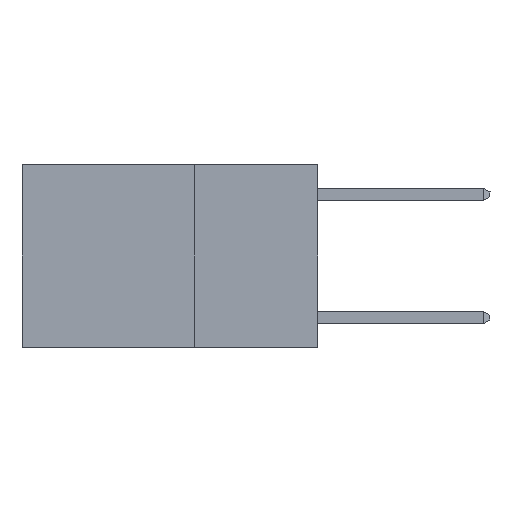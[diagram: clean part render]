
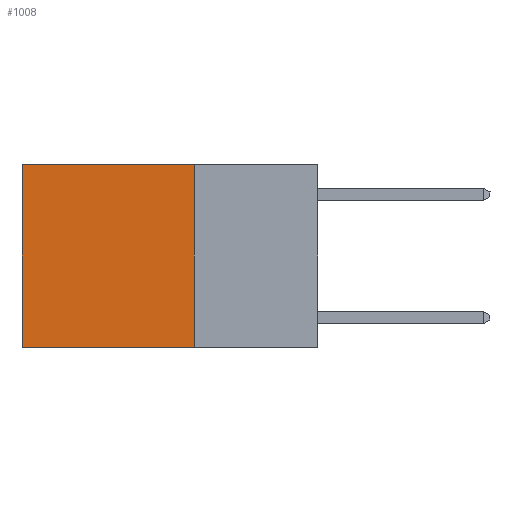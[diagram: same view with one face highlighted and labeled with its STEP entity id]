
A CAD part, left-side view. The second image highlights one B-rep face of the part: STEP entity #1008.
In plain terms, the highlighted planar face has unit normal (-1, 0, 0).
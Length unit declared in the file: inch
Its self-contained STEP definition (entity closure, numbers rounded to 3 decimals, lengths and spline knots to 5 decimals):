
#23 = ORIENTED_EDGE ( 'NONE', *, *, #8157, .T. ) ;
#970 = ORIENTED_EDGE ( 'NONE', *, *, #1598, .T. ) ;
#1008 = ADVANCED_FACE ( 'NONE', ( #7359 ), #7798, .F. ) ;
#1027 = LINE ( 'NONE', #3263, #15625 ) ;
#1598 = EDGE_CURVE ( 'NONE', #15399, #4673, #9685, .T. ) ;
#1655 = LINE ( 'NONE', #2238, #15828 ) ;
#2238 = CARTESIAN_POINT ( 'NONE',  ( 0.2625, 0.25, 0. ) ) ;
#2311 = CARTESIAN_POINT ( 'NONE',  ( 0.2625, 0.6, -0.37 ) ) ;
#2419 = DIRECTION ( 'NONE',  ( 0., 0., -1. ) ) ;
#3263 = CARTESIAN_POINT ( 'NONE',  ( 0.2625, 0.25, 0. ) ) ;
#4673 = VERTEX_POINT ( 'NONE', #2311 ) ;
#5084 = VECTOR ( 'NONE', #8416, 39.37008 ) ;
#5508 = LINE ( 'NONE', #9764, #5084 ) ;
#5667 = AXIS2_PLACEMENT_3D ( 'NONE', #12930, #12880, #9651 ) ;
#6391 = EDGE_LOOP ( 'NONE', ( #970, #12656, #12473, #23 ) ) ;
#6484 = CARTESIAN_POINT ( 'NONE',  ( 0.2625, 0.25, 0. ) ) ;
#6863 = VERTEX_POINT ( 'NONE', #14920 ) ;
#7359 = FACE_OUTER_BOUND ( 'NONE', #6391, .T. ) ;
#7798 = PLANE ( 'NONE',  #5667 ) ;
#7958 = EDGE_CURVE ( 'NONE', #13203, #6863, #1027, .T. ) ;
#8157 = EDGE_CURVE ( 'NONE', #13203, #15399, #1655, .T. ) ;
#8416 = DIRECTION ( 'NONE',  ( 0., 1., 0. ) ) ;
#8732 = DIRECTION ( 'NONE',  ( 0., 0., -1. ) ) ;
#9247 = CARTESIAN_POINT ( 'NONE',  ( 0.2625, 0.6, 0. ) ) ;
#9651 = DIRECTION ( 'NONE',  ( 0., 0., -1. ) ) ;
#9685 = LINE ( 'NONE', #9247, #16169 ) ;
#9764 = CARTESIAN_POINT ( 'NONE',  ( 0.2625, 0.25, -0.37 ) ) ;
#12473 = ORIENTED_EDGE ( 'NONE', *, *, #7958, .F. ) ;
#12656 = ORIENTED_EDGE ( 'NONE', *, *, #12793, .F. ) ;
#12793 = EDGE_CURVE ( 'NONE', #6863, #4673, #5508, .T. ) ;
#12880 = DIRECTION ( 'NONE',  ( 1., 0., 0. ) ) ;
#12930 = CARTESIAN_POINT ( 'NONE',  ( 0.2625, 0.25, 0. ) ) ;
#13203 = VERTEX_POINT ( 'NONE', #6484 ) ;
#14667 = DIRECTION ( 'NONE',  ( 0., 1., 0. ) ) ;
#14920 = CARTESIAN_POINT ( 'NONE',  ( 0.2625, 0.25, -0.37 ) ) ;
#15107 = CARTESIAN_POINT ( 'NONE',  ( 0.2625, 0.6, 0. ) ) ;
#15399 = VERTEX_POINT ( 'NONE', #15107 ) ;
#15625 = VECTOR ( 'NONE', #8732, 39.37008 ) ;
#15828 = VECTOR ( 'NONE', #14667, 39.37008 ) ;
#16169 = VECTOR ( 'NONE', #2419, 39.37008 ) ;
